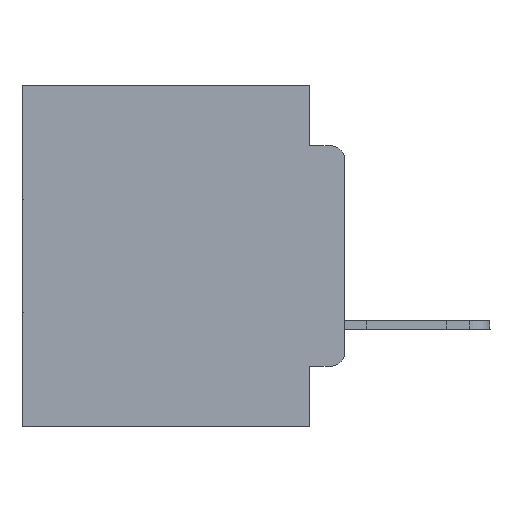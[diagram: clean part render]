
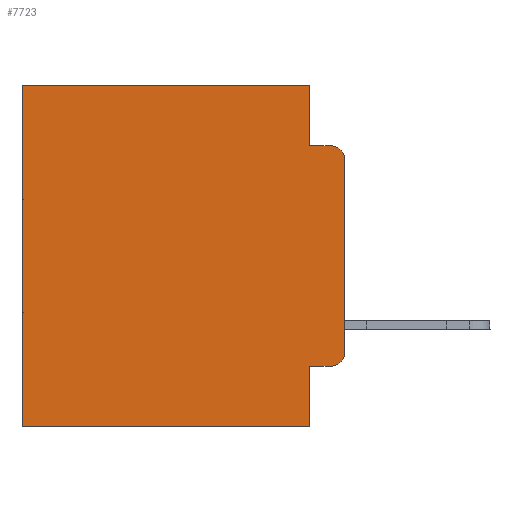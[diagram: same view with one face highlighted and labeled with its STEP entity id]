
A CAD part, left-side view. The second image highlights one B-rep face of the part: STEP entity #7723.
In plain terms, the highlighted planar face has unit normal (-1, 0, 0).
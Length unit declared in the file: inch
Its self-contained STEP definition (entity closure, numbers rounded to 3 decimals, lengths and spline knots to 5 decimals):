
#651 = VECTOR ( 'NONE', #3430, 39.37008 ) ;
#938 = ORIENTED_EDGE ( 'NONE', *, *, #15193, .T. ) ;
#952 = EDGE_CURVE ( 'NONE', #7758, #16243, #21026, .T. ) ;
#1074 = EDGE_CURVE ( 'NONE', #15728, #22945, #15075, .T. ) ;
#1800 = LINE ( 'NONE', #17919, #8973 ) ;
#2042 = VERTEX_POINT ( 'NONE', #25677 ) ;
#2430 = EDGE_CURVE ( 'NONE', #24637, #8701, #23002, .T. ) ;
#3340 = EDGE_CURVE ( 'NONE', #16402, #22945, #28088, .T. ) ;
#3430 = DIRECTION ( 'NONE',  ( 0., -1., 0. ) ) ;
#3809 = AXIS2_PLACEMENT_3D ( 'NONE', #20455, #24958, #19997 ) ;
#4191 = ORIENTED_EDGE ( 'NONE', *, *, #1074, .F. ) ;
#4502 = CARTESIAN_POINT ( 'NONE',  ( 0.298, 0.051, -0.0885 ) ) ;
#5042 = EDGE_LOOP ( 'NONE', ( #4191, #15189, #23659, #21441, #938, #23070, #8481, #8708, #19578, #24066 ) ) ;
#5724 = VERTEX_POINT ( 'NONE', #14421 ) ;
#6754 = CARTESIAN_POINT ( 'NONE',  ( 0.298, 0.051, 0. ) ) ;
#7015 = CARTESIAN_POINT ( 'NONE',  ( 0.298, 0.051, 0. ) ) ;
#7315 = DIRECTION ( 'NONE',  ( 0., 0., -1. ) ) ;
#7393 = FACE_OUTER_BOUND ( 'NONE', #5042, .T. ) ;
#7723 = ADVANCED_FACE ( 'NONE', ( #7393 ), #16830, .F. ) ;
#7758 = VERTEX_POINT ( 'NONE', #22415 ) ;
#8091 = CARTESIAN_POINT ( 'NONE',  ( 0.298, 0.051, -0.0885 ) ) ;
#8118 = CARTESIAN_POINT ( 'NONE',  ( 0.298, 0., 0. ) ) ;
#8280 = VECTOR ( 'NONE', #12301, 39.37008 ) ;
#8481 = ORIENTED_EDGE ( 'NONE', *, *, #8777, .F. ) ;
#8701 = VERTEX_POINT ( 'NONE', #29263 ) ;
#8708 = ORIENTED_EDGE ( 'NONE', *, *, #27906, .F. ) ;
#8777 = EDGE_CURVE ( 'NONE', #5724, #8701, #14990, .T. ) ;
#8973 = VECTOR ( 'NONE', #10793, 39.37008 ) ;
#9538 = VECTOR ( 'NONE', #7315, 39.37008 ) ;
#9606 = EDGE_CURVE ( 'NONE', #2042, #16402, #14766, .T. ) ;
#10459 = CARTESIAN_POINT ( 'NONE',  ( 0.298, 0.473, 0. ) ) ;
#10793 = DIRECTION ( 'NONE',  ( 0., 1., 0. ) ) ;
#11072 = VECTOR ( 'NONE', #21474, 39.37008 ) ;
#11092 = EDGE_CURVE ( 'NONE', #15728, #23190, #23695, .T. ) ;
#12301 = DIRECTION ( 'NONE',  ( 0., -1., 0. ) ) ;
#12546 = CARTESIAN_POINT ( 'NONE',  ( 0.298, 0.02, -0.4115 ) ) ;
#12863 = CARTESIAN_POINT ( 'NONE',  ( 0.298, 0.02, -0.0885 ) ) ;
#12876 = LINE ( 'NONE', #8091, #651 ) ;
#14421 = CARTESIAN_POINT ( 'NONE',  ( 0.298, 0.051, -0.5 ) ) ;
#14514 = DIRECTION ( 'NONE',  ( 0., 0., -1. ) ) ;
#14766 = LINE ( 'NONE', #28750, #8280 ) ;
#14778 = DIRECTION ( 'NONE',  ( 0., 0., -1. ) ) ;
#14990 = LINE ( 'NONE', #19525, #17627 ) ;
#15075 = LINE ( 'NONE', #8118, #17018 ) ;
#15189 = ORIENTED_EDGE ( 'NONE', *, *, #11092, .T. ) ;
#15193 = EDGE_CURVE ( 'NONE', #7758, #24637, #1800, .T. ) ;
#15728 = VERTEX_POINT ( 'NONE', #23154 ) ;
#16243 = VERTEX_POINT ( 'NONE', #4502 ) ;
#16306 = CARTESIAN_POINT ( 'NONE',  ( 0.298, 0., -0.3915 ) ) ;
#16402 = VERTEX_POINT ( 'NONE', #12546 ) ;
#16459 = DIRECTION ( 'NONE',  ( 0., 0., -1. ) ) ;
#16830 = PLANE ( 'NONE',  #30650 ) ;
#17018 = VECTOR ( 'NONE', #14778, 39.37008 ) ;
#17263 = EDGE_CURVE ( 'NONE', #16243, #23190, #12876, .T. ) ;
#17627 = VECTOR ( 'NONE', #22003, 39.37008 ) ;
#17919 = CARTESIAN_POINT ( 'NONE',  ( 0.298, 0., 0. ) ) ;
#19525 = CARTESIAN_POINT ( 'NONE',  ( 0.298, 0., -0.5 ) ) ;
#19578 = ORIENTED_EDGE ( 'NONE', *, *, #9606, .T. ) ;
#19997 = DIRECTION ( 'NONE',  ( 0., 0., -1. ) ) ;
#20369 = CARTESIAN_POINT ( 'NONE',  ( 0.298, 0.473, 0. ) ) ;
#20455 = CARTESIAN_POINT ( 'NONE',  ( 0.298, 0.02, -0.3915 ) ) ;
#21026 = LINE ( 'NONE', #6754, #11072 ) ;
#21441 = ORIENTED_EDGE ( 'NONE', *, *, #952, .F. ) ;
#21474 = DIRECTION ( 'NONE',  ( 0., 0., -1. ) ) ;
#21973 = DIRECTION ( 'NONE',  ( 1., 0., 0. ) ) ;
#22003 = DIRECTION ( 'NONE',  ( 0., 1., 0. ) ) ;
#22415 = CARTESIAN_POINT ( 'NONE',  ( 0.298, 0.051, 0. ) ) ;
#22945 = VERTEX_POINT ( 'NONE', #16306 ) ;
#23002 = LINE ( 'NONE', #20369, #26673 ) ;
#23070 = ORIENTED_EDGE ( 'NONE', *, *, #2430, .T. ) ;
#23154 = CARTESIAN_POINT ( 'NONE',  ( 0.298, 0., -0.1085 ) ) ;
#23190 = VERTEX_POINT ( 'NONE', #12863 ) ;
#23605 = CARTESIAN_POINT ( 'NONE',  ( 0.298, 0.02, -0.1085 ) ) ;
#23659 = ORIENTED_EDGE ( 'NONE', *, *, #17263, .F. ) ;
#23695 = CIRCLE ( 'NONE', #24684, 0.02 ) ;
#23904 = LINE ( 'NONE', #7015, #9538 ) ;
#24066 = ORIENTED_EDGE ( 'NONE', *, *, #3340, .T. ) ;
#24637 = VERTEX_POINT ( 'NONE', #10459 ) ;
#24684 = AXIS2_PLACEMENT_3D ( 'NONE', #23605, #28106, #16459 ) ;
#24958 = DIRECTION ( 'NONE',  ( -1., 0., 0. ) ) ;
#25677 = CARTESIAN_POINT ( 'NONE',  ( 0.298, 0.051, -0.4115 ) ) ;
#26315 = CARTESIAN_POINT ( 'NONE',  ( 0.298, 0., 0. ) ) ;
#26673 = VECTOR ( 'NONE', #30131, 39.37008 ) ;
#27906 = EDGE_CURVE ( 'NONE', #2042, #5724, #23904, .T. ) ;
#28088 = CIRCLE ( 'NONE', #3809, 0.02 ) ;
#28106 = DIRECTION ( 'NONE',  ( -1., 0., 0. ) ) ;
#28750 = CARTESIAN_POINT ( 'NONE',  ( 0.298, 0.051, -0.4115 ) ) ;
#29263 = CARTESIAN_POINT ( 'NONE',  ( 0.298, 0.473, -0.5 ) ) ;
#30131 = DIRECTION ( 'NONE',  ( 0., 0., -1. ) ) ;
#30650 = AXIS2_PLACEMENT_3D ( 'NONE', #26315, #21973, #14514 ) ;
